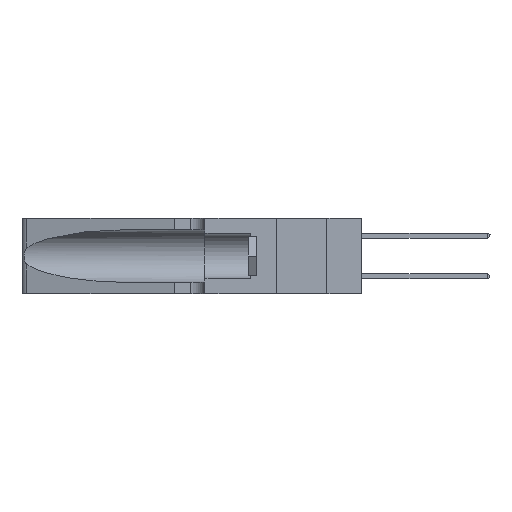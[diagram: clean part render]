
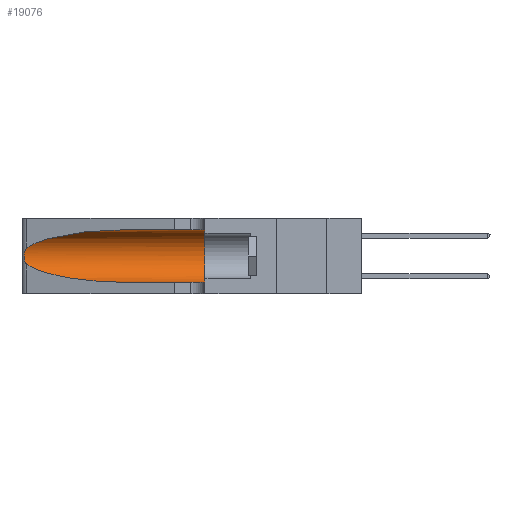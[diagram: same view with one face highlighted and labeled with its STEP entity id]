
A CAD part, left-side view. The second image highlights one B-rep face of the part: STEP entity #19076.
In plain terms, the highlighted cylindrical face has radius 3.308 mm (diameter 6.617 mm), a partial arc.
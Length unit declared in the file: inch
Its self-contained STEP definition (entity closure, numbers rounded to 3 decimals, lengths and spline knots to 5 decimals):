
#218 = EDGE_CURVE ( 'NONE', #8650, #5121, #3576, .T. ) ;
#1349 = CARTESIAN_POINT ( 'NONE',  ( 0.25787, 1.23484, 0.2124 ) ) ;
#2762 = EDGE_CURVE ( 'NONE', #21042, #5121, #6942, .T. ) ;
#2809 = ORIENTED_EDGE ( 'NONE', *, *, #17888, .F. ) ;
#3576 = CIRCLE ( 'NONE', #11848, 0.13025 ) ;
#3985 = DIRECTION ( 'NONE',  ( 0., -1., 0. ) ) ;
#4226 = CARTESIAN_POINT ( 'NONE',  ( 0.26018, 1.23835, 0.19895 ) ) ;
#5121 = VERTEX_POINT ( 'NONE', #16968 ) ;
#5777 = ORIENTED_EDGE ( 'NONE', *, *, #33135, .T. ) ;
#6338 = CARTESIAN_POINT ( 'NONE',  ( 0.2373, 1.15595, 0.08982 ) ) ;
#6534 = CARTESIAN_POINT ( 'NONE',  ( 0.2373, 1.15595, 0.28018 ) ) ;
#6942 = LINE ( 'NONE', #15198, #35407 ) ;
#7096 = CARTESIAN_POINT ( 'NONE',  ( 0.26075, 1.23896, 0.178 ) ) ;
#7486 = EDGE_CURVE ( 'NONE', #25648, #21042, #35329, .T. ) ;
#7494 = ORIENTED_EDGE ( 'NONE', *, *, #2762, .T. ) ;
#7781 = ORIENTED_EDGE ( 'NONE', *, *, #218, .F. ) ;
#8650 = VERTEX_POINT ( 'NONE', #27607 ) ;
#9144 = CARTESIAN_POINT ( 'NONE',  ( 0.18966, 0.96281, 0.31525 ) ) ;
#9277 = CARTESIAN_POINT ( 'NONE',  ( 0.1305, 0.72297, 0.31525 ) ) ;
#9825 = CARTESIAN_POINT ( 'NONE',  ( 0.25555, 1.22994, 0.2215 ) ) ;
#9943 = CARTESIAN_POINT ( 'NONE',  ( 0.25856, 1.23593, 0.16098 ) ) ;
#10035 = FACE_OUTER_BOUND ( 'NONE', #35132, .T. ) ;
#10381 = CARTESIAN_POINT ( 'NONE',  ( 0.25487, 1.22718, 0.14631 ) ) ;
#11097 = CARTESIAN_POINT ( 'NONE',  ( 0.25487, 1.22718, 0.22369 ) ) ;
#11433 = VECTOR ( 'NONE', #33698, 39.37008 ) ;
#11848 = AXIS2_PLACEMENT_3D ( 'NONE', #30298, #13871, #33039 ) ;
#12771 = CARTESIAN_POINT ( 'NONE',  ( 0.25639, 1.23186, 0.15144 ) ) ;
#13871 = DIRECTION ( 'NONE',  ( 0., 1., 0. ) ) ;
#14120 = VERTEX_POINT ( 'NONE', #11097 ) ;
#14818 = CARTESIAN_POINT ( 'NONE',  ( 0.1305, 0.72297, 0.05475 ) ) ;
#15198 = CARTESIAN_POINT ( 'NONE',  ( 0.1305, 1.61858, 0.05475 ) ) ;
#15556 = CARTESIAN_POINT ( 'NONE',  ( 0.25487, 1.22718, 0.14631 ) ) ;
#15692 = CYLINDRICAL_SURFACE ( 'NONE', #19675, 0.13025 ) ;
#16929 = VERTEX_POINT ( 'NONE', #26730 ) ;
#16968 = CARTESIAN_POINT ( 'NONE',  ( 0.1305, 0.35, 0.05475 ) ) ;
#17888 = EDGE_CURVE ( 'NONE', #16929, #8650, #33349, .T. ) ;
#18026 = DIRECTION ( 'NONE',  ( 0., -1., 0. ) ) ;
#18196 = CARTESIAN_POINT ( 'NONE',  ( 0.25639, 1.23184, 0.21858 ) ) ;
#18888 = ORIENTED_EDGE ( 'NONE', *, *, #7486, .T. ) ;
#19076 = ADVANCED_FACE ( 'NONE', ( #10035 ), #15692, .F. ) ;
#19675 = AXIS2_PLACEMENT_3D ( 'NONE', #31785, #18026, #20814 ) ;
#19947 = CARTESIAN_POINT ( 'NONE',  ( 0.1305, 1.61858, 0.31525 ) ) ;
#19996 = B_SPLINE_CURVE_WITH_KNOTS ( 'NONE', 3,
 ( #29125, #9825, #18196, #1349, #20994, #4226, #23754, #7096, #26495, #9943, #29244, #12771, #31963, #15556 ),
 .UNSPECIFIED., .F., .F.,
 ( 4, 2, 2, 2, 2, 2, 4 ),
 ( 0., 0.00027, 0.00053, 0.00107, 0.0016, 0.00187, 0.00214 ),
 .UNSPECIFIED. ) ;
#20814 = DIRECTION ( 'NONE',  ( 0., 0., -1. ) ) ;
#20994 = CARTESIAN_POINT ( 'NONE',  ( 0.25854, 1.2359, 0.20912 ) ) ;
#21042 = VERTEX_POINT ( 'NONE', #31792 ) ;
#23754 = CARTESIAN_POINT ( 'NONE',  ( 0.26075, 1.23896, 0.19203 ) ) ;
#25648 = VERTEX_POINT ( 'NONE', #10381 ) ;
#25767 = CARTESIAN_POINT ( 'NONE',  ( 0.18966, 0.96281, 0.05475 ) ) ;
#25948 = CARTESIAN_POINT ( 'NONE',  ( 0.25487, 1.22718, 0.22369 ) ) ;
#26380 =( BOUNDED_CURVE ( )  B_SPLINE_CURVE ( 3, ( #9277, #9144, #6534, #25948 ),
 .UNSPECIFIED., .F., .T. ) 
 B_SPLINE_CURVE_WITH_KNOTS ( ( 4, 4 ),
 ( 1.5708, 2.84003 ),
 .UNSPECIFIED. ) 
 CURVE ( )  GEOMETRIC_REPRESENTATION_ITEM ( )  RATIONAL_B_SPLINE_CURVE ( ( 1., 0.87, 0.87, 1. ) ) 
 REPRESENTATION_ITEM ( '' )  );
#26495 = CARTESIAN_POINT ( 'NONE',  ( 0.26017, 1.23833, 0.17102 ) ) ;
#26730 = CARTESIAN_POINT ( 'NONE',  ( 0.1305, 0.72297, 0.31525 ) ) ;
#27607 = CARTESIAN_POINT ( 'NONE',  ( 0.1305, 0.35, 0.31525 ) ) ;
#27778 = ORIENTED_EDGE ( 'NONE', *, *, #30297, .T. ) ;
#29125 = CARTESIAN_POINT ( 'NONE',  ( 0.25487, 1.22718, 0.22369 ) ) ;
#29244 = CARTESIAN_POINT ( 'NONE',  ( 0.25789, 1.23486, 0.15765 ) ) ;
#30297 = EDGE_CURVE ( 'NONE', #16929, #14120, #26380, .T. ) ;
#30298 = CARTESIAN_POINT ( 'NONE',  ( 0.1305, 0.35, 0.185 ) ) ;
#31233 = CARTESIAN_POINT ( 'NONE',  ( 0.25487, 1.22718, 0.14631 ) ) ;
#31785 = CARTESIAN_POINT ( 'NONE',  ( 0.1305, 1.61858, 0.185 ) ) ;
#31792 = CARTESIAN_POINT ( 'NONE',  ( 0.1305, 0.72297, 0.05475 ) ) ;
#31963 = CARTESIAN_POINT ( 'NONE',  ( 0.25555, 1.22993, 0.14849 ) ) ;
#33039 = DIRECTION ( 'NONE',  ( 0., 0., 1. ) ) ;
#33135 = EDGE_CURVE ( 'NONE', #14120, #25648, #19996, .T. ) ;
#33349 = LINE ( 'NONE', #19947, #11433 ) ;
#33698 = DIRECTION ( 'NONE',  ( 0., -1., 0. ) ) ;
#35132 = EDGE_LOOP ( 'NONE', ( #27778, #5777, #18888, #7494, #7781, #2809 ) ) ;
#35329 =( BOUNDED_CURVE ( )  B_SPLINE_CURVE ( 3, ( #31233, #6338, #25767, #14818 ),
 .UNSPECIFIED., .F., .T. ) 
 B_SPLINE_CURVE_WITH_KNOTS ( ( 4, 4 ),
 ( 3.44316, 4.71239 ),
 .UNSPECIFIED. ) 
 CURVE ( )  GEOMETRIC_REPRESENTATION_ITEM ( )  RATIONAL_B_SPLINE_CURVE ( ( 1., 0.87, 0.87, 1. ) ) 
 REPRESENTATION_ITEM ( '' )  );
#35407 = VECTOR ( 'NONE', #3985, 39.37008 ) ;
